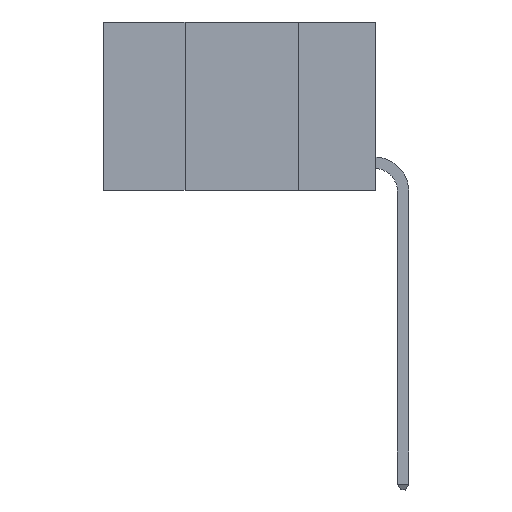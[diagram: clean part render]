
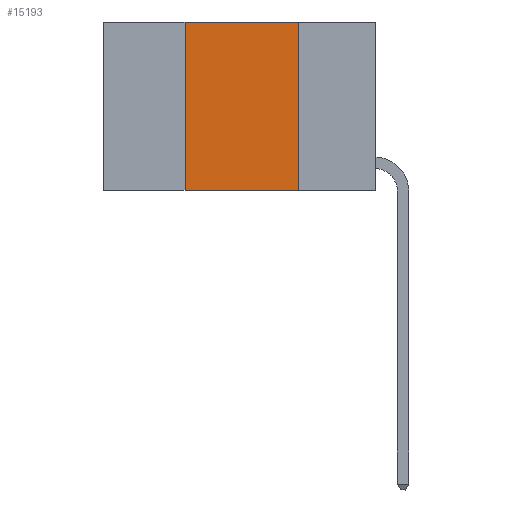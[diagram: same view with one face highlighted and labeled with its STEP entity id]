
A CAD part, left-side view. The second image highlights one B-rep face of the part: STEP entity #15193.
In plain terms, the highlighted planar face has unit normal (-1, 0, 0).
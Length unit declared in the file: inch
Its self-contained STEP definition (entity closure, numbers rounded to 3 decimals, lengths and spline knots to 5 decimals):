
#24 = DIRECTION ( 'NONE',  ( 0., 0., -1. ) ) ;
#385 = ORIENTED_EDGE ( 'NONE', *, *, #15899, .F. ) ;
#553 = LINE ( 'NONE', #9718, #17899 ) ;
#761 = ORIENTED_EDGE ( 'NONE', *, *, #15122, .F. ) ;
#2323 = CARTESIAN_POINT ( 'NONE',  ( 0., 0.17, -0.37 ) ) ;
#3620 = LINE ( 'NONE', #10683, #25002 ) ;
#4002 = ORIENTED_EDGE ( 'NONE', *, *, #16582, .F. ) ;
#4275 = DIRECTION ( 'NONE',  ( 0., 0., 1. ) ) ;
#4902 = VERTEX_POINT ( 'NONE', #7099 ) ;
#5115 = VECTOR ( 'NONE', #15443, 39.37008 ) ;
#7099 = CARTESIAN_POINT ( 'NONE',  ( 0., 0.42, 0. ) ) ;
#7378 = FACE_OUTER_BOUND ( 'NONE', #24874, .T. ) ;
#8482 = VERTEX_POINT ( 'NONE', #2323 ) ;
#9336 = EDGE_CURVE ( 'NONE', #25697, #8482, #553, .T. ) ;
#9463 = VECTOR ( 'NONE', #19242, 39.37008 ) ;
#9718 = CARTESIAN_POINT ( 'NONE',  ( 0., 0.6, -0.37 ) ) ;
#9874 = AXIS2_PLACEMENT_3D ( 'NONE', #23692, #13135, #24 ) ;
#10683 = CARTESIAN_POINT ( 'NONE',  ( 0., 0.42, 0. ) ) ;
#13135 = DIRECTION ( 'NONE',  ( 1., 0., 0. ) ) ;
#13385 = CARTESIAN_POINT ( 'NONE',  ( 0., 0.6, 0. ) ) ;
#13492 = ORIENTED_EDGE ( 'NONE', *, *, #9336, .T. ) ;
#15122 = EDGE_CURVE ( 'NONE', #25697, #4902, #3620, .T. ) ;
#15193 = ADVANCED_FACE ( 'NONE', ( #7378 ), #19491, .F. ) ;
#15443 = DIRECTION ( 'NONE',  ( 0., -1., 0. ) ) ;
#15896 = LINE ( 'NONE', #17108, #9463 ) ;
#15899 = EDGE_CURVE ( 'NONE', #4902, #21652, #23466, .T. ) ;
#16582 = EDGE_CURVE ( 'NONE', #21652, #8482, #15896, .T. ) ;
#17108 = CARTESIAN_POINT ( 'NONE',  ( 0., 0.17, 0. ) ) ;
#17899 = VECTOR ( 'NONE', #22499, 39.37008 ) ;
#19242 = DIRECTION ( 'NONE',  ( 0., 0., -1. ) ) ;
#19491 = PLANE ( 'NONE',  #9874 ) ;
#21652 = VERTEX_POINT ( 'NONE', #27342 ) ;
#22499 = DIRECTION ( 'NONE',  ( 0., -1., 0. ) ) ;
#23466 = LINE ( 'NONE', #13385, #5115 ) ;
#23692 = CARTESIAN_POINT ( 'NONE',  ( 0., 0.6, 0. ) ) ;
#24874 = EDGE_LOOP ( 'NONE', ( #4002, #385, #761, #13492 ) ) ;
#25002 = VECTOR ( 'NONE', #4275, 39.37008 ) ;
#25242 = CARTESIAN_POINT ( 'NONE',  ( 0., 0.42, -0.37 ) ) ;
#25697 = VERTEX_POINT ( 'NONE', #25242 ) ;
#27342 = CARTESIAN_POINT ( 'NONE',  ( 0., 0.17, 0. ) ) ;
